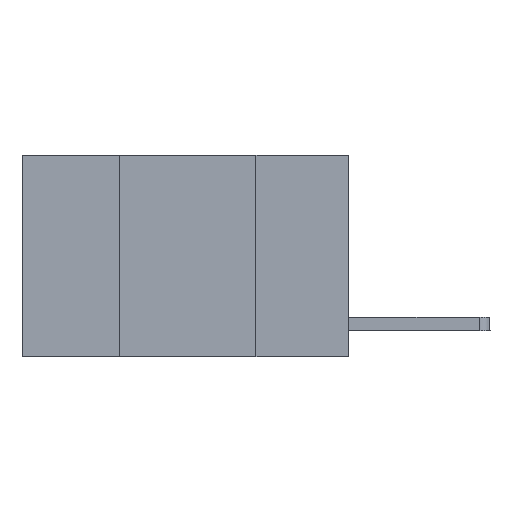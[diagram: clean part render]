
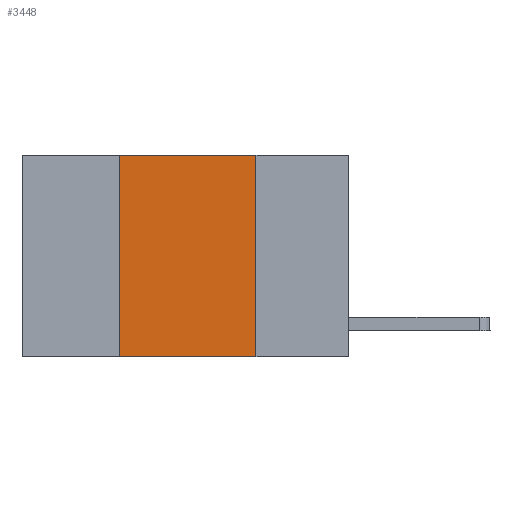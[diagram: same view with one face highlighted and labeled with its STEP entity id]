
A CAD part, left-side view. The second image highlights one B-rep face of the part: STEP entity #3448.
In plain terms, the highlighted planar face has unit normal (-1, 0, 0).
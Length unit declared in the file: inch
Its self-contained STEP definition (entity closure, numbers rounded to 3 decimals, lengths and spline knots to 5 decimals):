
#1038 = VECTOR ( 'NONE', #3094, 39.37008 ) ;
#1341 = DIRECTION ( 'NONE',  ( 0., 0., -1. ) ) ;
#1438 = ORIENTED_EDGE ( 'NONE', *, *, #6797, .F. ) ;
#1647 = VERTEX_POINT ( 'NONE', #2173 ) ;
#1829 = CARTESIAN_POINT ( 'NONE',  ( 0., 0.6, -0.37 ) ) ;
#2173 = CARTESIAN_POINT ( 'NONE',  ( 0., 0.17, 0. ) ) ;
#2206 = EDGE_CURVE ( 'NONE', #1647, #5927, #8353, .T. ) ;
#2225 = VECTOR ( 'NONE', #8457, 39.37008 ) ;
#2365 = CARTESIAN_POINT ( 'NONE',  ( 0., 0.17, -0.37 ) ) ;
#2510 = ORIENTED_EDGE ( 'NONE', *, *, #2206, .F. ) ;
#2711 = DIRECTION ( 'NONE',  ( 1., 0., 0. ) ) ;
#2895 = EDGE_LOOP ( 'NONE', ( #2510, #8333, #1438, #8279 ) ) ;
#3047 = DIRECTION ( 'NONE',  ( 0., 0., 1. ) ) ;
#3094 = DIRECTION ( 'NONE',  ( 0., 0., -1. ) ) ;
#3188 = LINE ( 'NONE', #1829, #2225 ) ;
#3448 = ADVANCED_FACE ( 'NONE', ( #6479 ), #5187, .F. ) ;
#3456 = CARTESIAN_POINT ( 'NONE',  ( 0., 0.17, 0. ) ) ;
#3504 = LINE ( 'NONE', #3895, #3513 ) ;
#3513 = VECTOR ( 'NONE', #3855, 39.37008 ) ;
#3615 = AXIS2_PLACEMENT_3D ( 'NONE', #5990, #2711, #1341 ) ;
#3698 = CARTESIAN_POINT ( 'NONE',  ( 0., 0.42, 0. ) ) ;
#3855 = DIRECTION ( 'NONE',  ( 0., -1., 0. ) ) ;
#3895 = CARTESIAN_POINT ( 'NONE',  ( 0., 0.6, 0. ) ) ;
#4453 = LINE ( 'NONE', #3698, #8065 ) ;
#5152 = VERTEX_POINT ( 'NONE', #6021 ) ;
#5187 = PLANE ( 'NONE',  #3615 ) ;
#5722 = EDGE_CURVE ( 'NONE', #6090, #1647, #3504, .T. ) ;
#5927 = VERTEX_POINT ( 'NONE', #2365 ) ;
#5990 = CARTESIAN_POINT ( 'NONE',  ( 0., 0.6, 0. ) ) ;
#6021 = CARTESIAN_POINT ( 'NONE',  ( 0., 0.42, -0.37 ) ) ;
#6090 = VERTEX_POINT ( 'NONE', #8378 ) ;
#6479 = FACE_OUTER_BOUND ( 'NONE', #2895, .T. ) ;
#6529 = EDGE_CURVE ( 'NONE', #5152, #5927, #3188, .T. ) ;
#6797 = EDGE_CURVE ( 'NONE', #5152, #6090, #4453, .T. ) ;
#8065 = VECTOR ( 'NONE', #3047, 39.37008 ) ;
#8279 = ORIENTED_EDGE ( 'NONE', *, *, #6529, .T. ) ;
#8333 = ORIENTED_EDGE ( 'NONE', *, *, #5722, .F. ) ;
#8353 = LINE ( 'NONE', #3456, #1038 ) ;
#8378 = CARTESIAN_POINT ( 'NONE',  ( 0., 0.42, 0. ) ) ;
#8457 = DIRECTION ( 'NONE',  ( 0., -1., 0. ) ) ;
